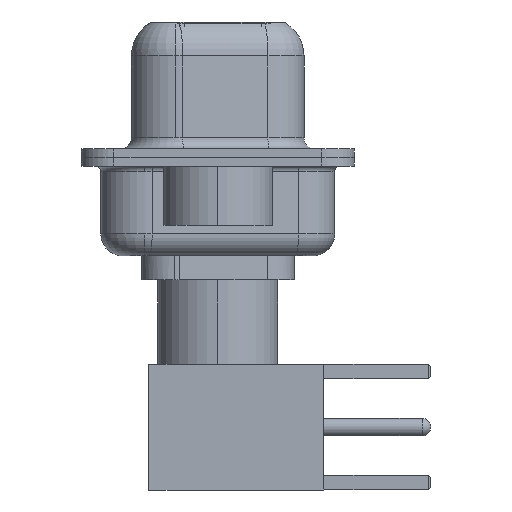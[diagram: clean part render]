
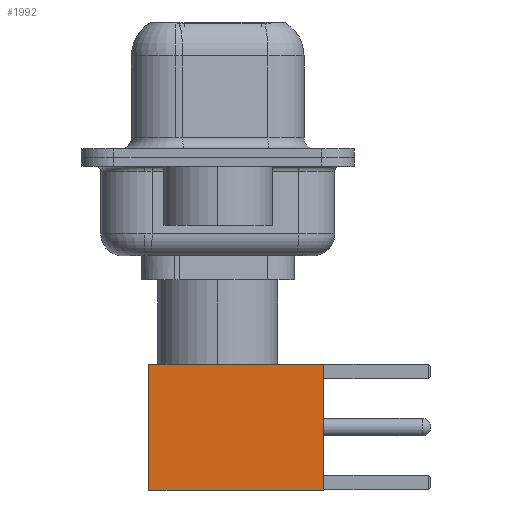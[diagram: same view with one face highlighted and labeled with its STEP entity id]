
A CAD part, left-side view. The second image highlights one B-rep face of the part: STEP entity #1992.
In plain terms, the highlighted face is planar.
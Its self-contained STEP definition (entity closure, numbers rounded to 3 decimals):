
#564 = PLANE ( 'NONE',  #14026 ) ;
#1992 = ADVANCED_FACE ( 'NONE', ( #2018 ), #564, .T. ) ;
#2018 = FACE_OUTER_BOUND ( 'NONE', #13536, .T. ) ;
#2028 = EDGE_CURVE ( 'NONE', #11911, #4701, #3045, .T. ) ;
#2407 = CARTESIAN_POINT ( 'NONE',  ( 0., 2.875, 0. ) ) ;
#2446 = EDGE_CURVE ( 'NONE', #11911, #15174, #12102, .T. ) ;
#3045 = LINE ( 'NONE', #13508, #9933 ) ;
#3761 = CARTESIAN_POINT ( 'NONE',  ( -2.875, 2.875, 0. ) ) ;
#3860 = VECTOR ( 'NONE', #4315, 1000. ) ;
#4046 = EDGE_CURVE ( 'NONE', #15174, #12635, #10123, .T. ) ;
#4315 = DIRECTION ( 'NONE',  ( 0., 0., -1. ) ) ;
#4418 = CARTESIAN_POINT ( 'NONE',  ( 2.875, 2.875, 8. ) ) ;
#4701 = VERTEX_POINT ( 'NONE', #6929 ) ;
#5291 = CARTESIAN_POINT ( 'NONE',  ( 2.875, 2.875, 0. ) ) ;
#5695 = CARTESIAN_POINT ( 'NONE',  ( 2.875, 2.875, 0. ) ) ;
#5768 = ORIENTED_EDGE ( 'NONE', *, *, #15201, .F. ) ;
#5901 = DIRECTION ( 'NONE',  ( 0., 1., 0. ) ) ;
#6929 = CARTESIAN_POINT ( 'NONE',  ( -2.875, 2.875, 8. ) ) ;
#7230 = DIRECTION ( 'NONE',  ( 0., 0., -1. ) ) ;
#7233 = CARTESIAN_POINT ( 'NONE',  ( -2.875, 2.875, 0. ) ) ;
#7252 = CARTESIAN_POINT ( 'NONE',  ( 2.875, 2.875, 0. ) ) ;
#7356 = ORIENTED_EDGE ( 'NONE', *, *, #4046, .T. ) ;
#7645 = DIRECTION ( 'NONE',  ( -1., 0., 0. ) ) ;
#8351 = LINE ( 'NONE', #7233, #3860 ) ;
#8621 = DIRECTION ( 'NONE',  ( -1., 0., 0. ) ) ;
#9277 = VECTOR ( 'NONE', #7645, 1000. ) ;
#9933 = VECTOR ( 'NONE', #8621, 1000. ) ;
#10123 = LINE ( 'NONE', #2407, #9277 ) ;
#11911 = VERTEX_POINT ( 'NONE', #4418 ) ;
#12102 = LINE ( 'NONE', #5695, #16260 ) ;
#12635 = VERTEX_POINT ( 'NONE', #3761 ) ;
#13508 = CARTESIAN_POINT ( 'NONE',  ( 0., 2.875, 8. ) ) ;
#13536 = EDGE_LOOP ( 'NONE', ( #13827, #7356, #5768, #14214 ) ) ;
#13827 = ORIENTED_EDGE ( 'NONE', *, *, #2446, .T. ) ;
#14026 = AXIS2_PLACEMENT_3D ( 'NONE', #7252, #5901, #14967 ) ;
#14214 = ORIENTED_EDGE ( 'NONE', *, *, #2028, .F. ) ;
#14967 = DIRECTION ( 'NONE',  ( 0., 0., 1. ) ) ;
#15174 = VERTEX_POINT ( 'NONE', #5291 ) ;
#15201 = EDGE_CURVE ( 'NONE', #4701, #12635, #8351, .T. ) ;
#16260 = VECTOR ( 'NONE', #7230, 1000. ) ;
